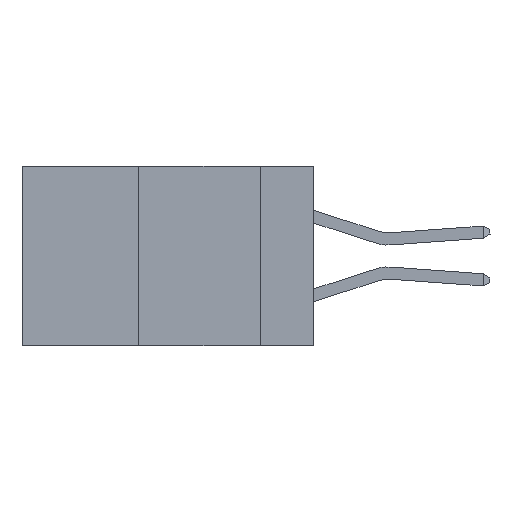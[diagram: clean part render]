
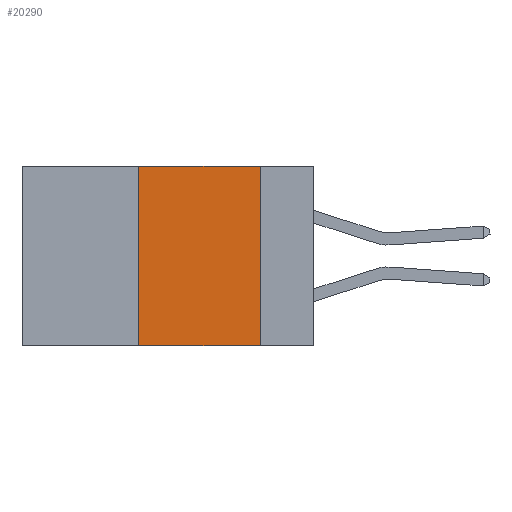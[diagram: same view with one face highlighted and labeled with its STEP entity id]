
A CAD part, left-side view. The second image highlights one B-rep face of the part: STEP entity #20290.
In plain terms, the highlighted planar face has unit normal (-1, 0, 0).
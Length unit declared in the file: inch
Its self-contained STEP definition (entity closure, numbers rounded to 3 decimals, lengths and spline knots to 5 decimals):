
#59 = VERTEX_POINT ( 'NONE', #2979 ) ;
#147 = EDGE_CURVE ( 'NONE', #9291, #14203, #3192, .T. ) ;
#610 = CARTESIAN_POINT ( 'NONE',  ( 0., 0.11, 0. ) ) ;
#1855 = CARTESIAN_POINT ( 'NONE',  ( 0., 0.6, 0. ) ) ;
#2291 = DIRECTION ( 'NONE',  ( 0., 0., -1. ) ) ;
#2979 = CARTESIAN_POINT ( 'NONE',  ( 0., 0.11, -0.37 ) ) ;
#3122 = CARTESIAN_POINT ( 'NONE',  ( 0., 0.36, 0. ) ) ;
#3192 = LINE ( 'NONE', #19967, #13411 ) ;
#3292 = FACE_OUTER_BOUND ( 'NONE', #19135, .T. ) ;
#4161 = LINE ( 'NONE', #610, #10462 ) ;
#6630 = CARTESIAN_POINT ( 'NONE',  ( 0., 0.11, 0. ) ) ;
#7567 = DIRECTION ( 'NONE',  ( 0., -1., 0. ) ) ;
#8493 = CARTESIAN_POINT ( 'NONE',  ( 0., 0.6, 0. ) ) ;
#8814 = VERTEX_POINT ( 'NONE', #6630 ) ;
#9291 = VERTEX_POINT ( 'NONE', #13590 ) ;
#9497 = EDGE_CURVE ( 'NONE', #9291, #59, #12769, .T. ) ;
#10084 = PLANE ( 'NONE',  #11246 ) ;
#10462 = VECTOR ( 'NONE', #16145, 39.37008 ) ;
#10476 = ORIENTED_EDGE ( 'NONE', *, *, #15742, .F. ) ;
#10885 = CARTESIAN_POINT ( 'NONE',  ( 0., 0.6, -0.37 ) ) ;
#11246 = AXIS2_PLACEMENT_3D ( 'NONE', #1855, #18724, #2291 ) ;
#12045 = EDGE_CURVE ( 'NONE', #14203, #8814, #19324, .T. ) ;
#12769 = LINE ( 'NONE', #10885, #15214 ) ;
#13411 = VECTOR ( 'NONE', #14969, 39.37008 ) ;
#13590 = CARTESIAN_POINT ( 'NONE',  ( 0., 0.36, -0.37 ) ) ;
#14203 = VERTEX_POINT ( 'NONE', #3122 ) ;
#14969 = DIRECTION ( 'NONE',  ( 0., 0., 1. ) ) ;
#15214 = VECTOR ( 'NONE', #17969, 39.37008 ) ;
#15742 = EDGE_CURVE ( 'NONE', #8814, #59, #4161, .T. ) ;
#16145 = DIRECTION ( 'NONE',  ( 0., 0., -1. ) ) ;
#16929 = ORIENTED_EDGE ( 'NONE', *, *, #12045, .F. ) ;
#17113 = VECTOR ( 'NONE', #7567, 39.37008 ) ;
#17969 = DIRECTION ( 'NONE',  ( 0., -1., 0. ) ) ;
#18724 = DIRECTION ( 'NONE',  ( 1., 0., 0. ) ) ;
#18930 = ORIENTED_EDGE ( 'NONE', *, *, #147, .F. ) ;
#19135 = EDGE_LOOP ( 'NONE', ( #10476, #16929, #18930, #21102 ) ) ;
#19324 = LINE ( 'NONE', #8493, #17113 ) ;
#19967 = CARTESIAN_POINT ( 'NONE',  ( 0., 0.36, 0. ) ) ;
#20290 = ADVANCED_FACE ( 'NONE', ( #3292 ), #10084, .F. ) ;
#21102 = ORIENTED_EDGE ( 'NONE', *, *, #9497, .T. ) ;
